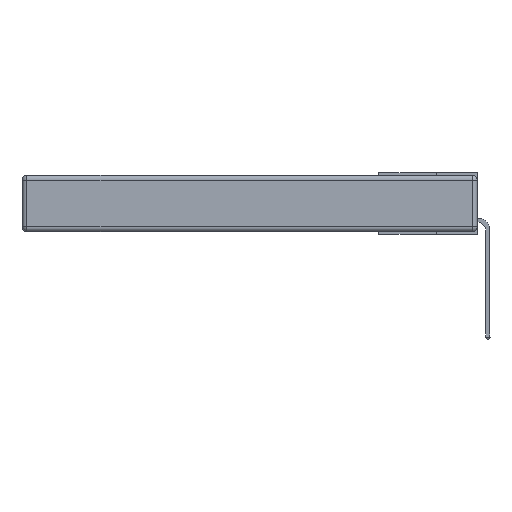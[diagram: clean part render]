
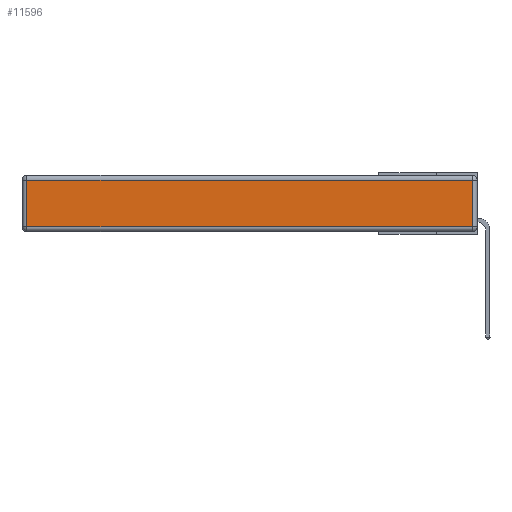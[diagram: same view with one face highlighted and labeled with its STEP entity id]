
A CAD part, left-side view. The second image highlights one B-rep face of the part: STEP entity #11596.
In plain terms, the highlighted planar face has unit normal (-1, 0, 0).
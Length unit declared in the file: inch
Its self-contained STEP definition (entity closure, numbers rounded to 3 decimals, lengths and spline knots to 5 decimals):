
#1028 = ORIENTED_EDGE ( 'NONE', *, *, #25812, .T. ) ;
#1188 = VERTEX_POINT ( 'NONE', #22827 ) ;
#1647 = CARTESIAN_POINT ( 'NONE',  ( 0., 0.03, -0.03 ) ) ;
#2849 = DIRECTION ( 'NONE',  ( -1., 0., 0. ) ) ;
#2861 = VECTOR ( 'NONE', #6744, 39.37008 ) ;
#2934 = DIRECTION ( 'NONE',  ( 0., 0., 1. ) ) ;
#3886 = EDGE_CURVE ( 'NONE', #1188, #5057, #12243, .T. ) ;
#4480 = EDGE_CURVE ( 'NONE', #9415, #9516, #19287, .T. ) ;
#5057 = VERTEX_POINT ( 'NONE', #23790 ) ;
#6744 = DIRECTION ( 'NONE',  ( 0., 0., 1. ) ) ;
#6940 = PLANE ( 'NONE',  #16327 ) ;
#8888 = VECTOR ( 'NONE', #23341, 39.37008 ) ;
#9415 = VERTEX_POINT ( 'NONE', #11839 ) ;
#9516 = VERTEX_POINT ( 'NONE', #1647 ) ;
#10395 = ORIENTED_EDGE ( 'NONE', *, *, #3886, .T. ) ;
#11596 = ADVANCED_FACE ( 'NONE', ( #18740 ), #6940, .T. ) ;
#11839 = CARTESIAN_POINT ( 'NONE',  ( 0., 0.03, -0.313 ) ) ;
#12243 = LINE ( 'NONE', #21165, #20791 ) ;
#14095 = LINE ( 'NONE', #15679, #18825 ) ;
#14293 = LINE ( 'NONE', #15627, #8888 ) ;
#15627 = CARTESIAN_POINT ( 'NONE',  ( 0., 0., -0.313 ) ) ;
#15679 = CARTESIAN_POINT ( 'NONE',  ( 0., 2.75, -0.03 ) ) ;
#16327 = AXIS2_PLACEMENT_3D ( 'NONE', #18913, #2849, #2934 ) ;
#17698 = DIRECTION ( 'NONE',  ( 0., 1., 0. ) ) ;
#18740 = FACE_OUTER_BOUND ( 'NONE', #20131, .T. ) ;
#18825 = VECTOR ( 'NONE', #17698, 39.37008 ) ;
#18882 = CARTESIAN_POINT ( 'NONE',  ( 0., 0.03, -0.343 ) ) ;
#18913 = CARTESIAN_POINT ( 'NONE',  ( 0., 0., -0.343 ) ) ;
#19287 = LINE ( 'NONE', #18882, #2861 ) ;
#20131 = EDGE_LOOP ( 'NONE', ( #1028, #23514, #26037, #10395 ) ) ;
#20791 = VECTOR ( 'NONE', #25012, 39.37008 ) ;
#21165 = CARTESIAN_POINT ( 'NONE',  ( 0., 2.72, -0.343 ) ) ;
#22827 = CARTESIAN_POINT ( 'NONE',  ( 0., 2.72, -0.03 ) ) ;
#23316 = EDGE_CURVE ( 'NONE', #9516, #1188, #14095, .T. ) ;
#23341 = DIRECTION ( 'NONE',  ( 0., -1., 0. ) ) ;
#23514 = ORIENTED_EDGE ( 'NONE', *, *, #4480, .T. ) ;
#23790 = CARTESIAN_POINT ( 'NONE',  ( 0., 2.72, -0.313 ) ) ;
#25012 = DIRECTION ( 'NONE',  ( 0., 0., -1. ) ) ;
#25812 = EDGE_CURVE ( 'NONE', #5057, #9415, #14293, .T. ) ;
#26037 = ORIENTED_EDGE ( 'NONE', *, *, #23316, .T. ) ;
